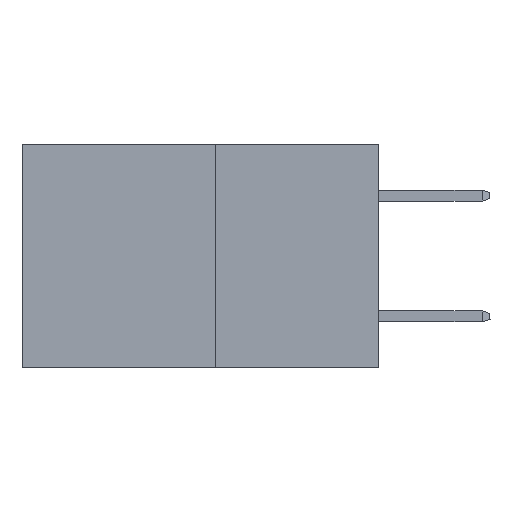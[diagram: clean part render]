
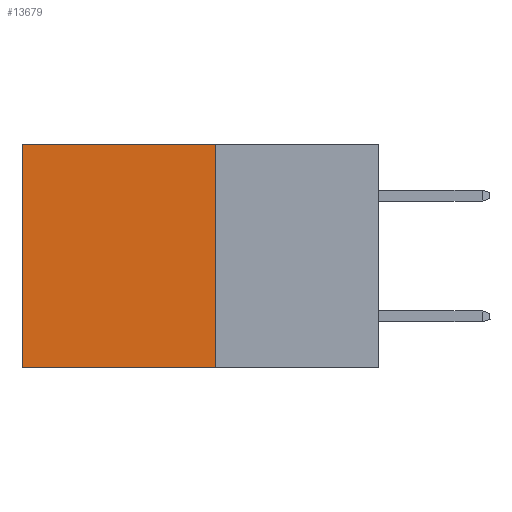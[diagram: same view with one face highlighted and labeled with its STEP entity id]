
A CAD part, left-side view. The second image highlights one B-rep face of the part: STEP entity #13679.
In plain terms, the highlighted planar face has unit normal (-1, 0, 0).
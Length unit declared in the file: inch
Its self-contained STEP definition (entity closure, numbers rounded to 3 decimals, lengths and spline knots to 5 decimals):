
#189 = VERTEX_POINT ( 'NONE', #13790 ) ;
#796 = CARTESIAN_POINT ( 'NONE',  ( 0.277, 0.27, -0.37 ) ) ;
#1371 = VERTEX_POINT ( 'NONE', #10742 ) ;
#1406 = CARTESIAN_POINT ( 'NONE',  ( 0.277, 0.27, 0. ) ) ;
#1707 = FACE_OUTER_BOUND ( 'NONE', #4975, .T. ) ;
#1789 = DIRECTION ( 'NONE',  ( 0., 1., 0. ) ) ;
#3337 = DIRECTION ( 'NONE',  ( 0., 0., -1. ) ) ;
#3413 = EDGE_CURVE ( 'NONE', #1371, #11376, #11578, .T. ) ;
#3772 = DIRECTION ( 'NONE',  ( 0., 0., -1. ) ) ;
#4718 = LINE ( 'NONE', #1406, #9919 ) ;
#4975 = EDGE_LOOP ( 'NONE', ( #12893, #12856, #10005, #11272 ) ) ;
#5133 = DIRECTION ( 'NONE',  ( 0., 1., 0. ) ) ;
#5683 = LINE ( 'NONE', #12692, #11178 ) ;
#5696 = PLANE ( 'NONE',  #12005 ) ;
#6938 = EDGE_CURVE ( 'NONE', #8357, #1371, #5683, .T. ) ;
#7305 = CARTESIAN_POINT ( 'NONE',  ( 0.277, 0.59, -0.37 ) ) ;
#7478 = VECTOR ( 'NONE', #3772, 39.37008 ) ;
#7608 = CARTESIAN_POINT ( 'NONE',  ( 0.277, 0.27, 0. ) ) ;
#7989 = DIRECTION ( 'NONE',  ( 0., 0., -1. ) ) ;
#8357 = VERTEX_POINT ( 'NONE', #7608 ) ;
#9040 = CARTESIAN_POINT ( 'NONE',  ( 0.277, 0.27, -0.37 ) ) ;
#9919 = VECTOR ( 'NONE', #5133, 39.37008 ) ;
#10005 = ORIENTED_EDGE ( 'NONE', *, *, #6938, .F. ) ;
#10121 = DIRECTION ( 'NONE',  ( 1., 0., 0. ) ) ;
#10398 = EDGE_CURVE ( 'NONE', #8357, #189, #4718, .T. ) ;
#10742 = CARTESIAN_POINT ( 'NONE',  ( 0.277, 0.27, -0.37 ) ) ;
#11178 = VECTOR ( 'NONE', #7989, 39.37008 ) ;
#11272 = ORIENTED_EDGE ( 'NONE', *, *, #10398, .T. ) ;
#11376 = VERTEX_POINT ( 'NONE', #11965 ) ;
#11578 = LINE ( 'NONE', #9040, #13376 ) ;
#11965 = CARTESIAN_POINT ( 'NONE',  ( 0.277, 0.59, -0.37 ) ) ;
#12005 = AXIS2_PLACEMENT_3D ( 'NONE', #796, #10121, #3337 ) ;
#12692 = CARTESIAN_POINT ( 'NONE',  ( 0.277, 0.27, -0.37 ) ) ;
#12856 = ORIENTED_EDGE ( 'NONE', *, *, #3413, .F. ) ;
#12893 = ORIENTED_EDGE ( 'NONE', *, *, #13996, .T. ) ;
#13110 = LINE ( 'NONE', #7305, #7478 ) ;
#13376 = VECTOR ( 'NONE', #1789, 39.37008 ) ;
#13679 = ADVANCED_FACE ( 'NONE', ( #1707 ), #5696, .F. ) ;
#13790 = CARTESIAN_POINT ( 'NONE',  ( 0.277, 0.59, 0. ) ) ;
#13996 = EDGE_CURVE ( 'NONE', #189, #11376, #13110, .T. ) ;
